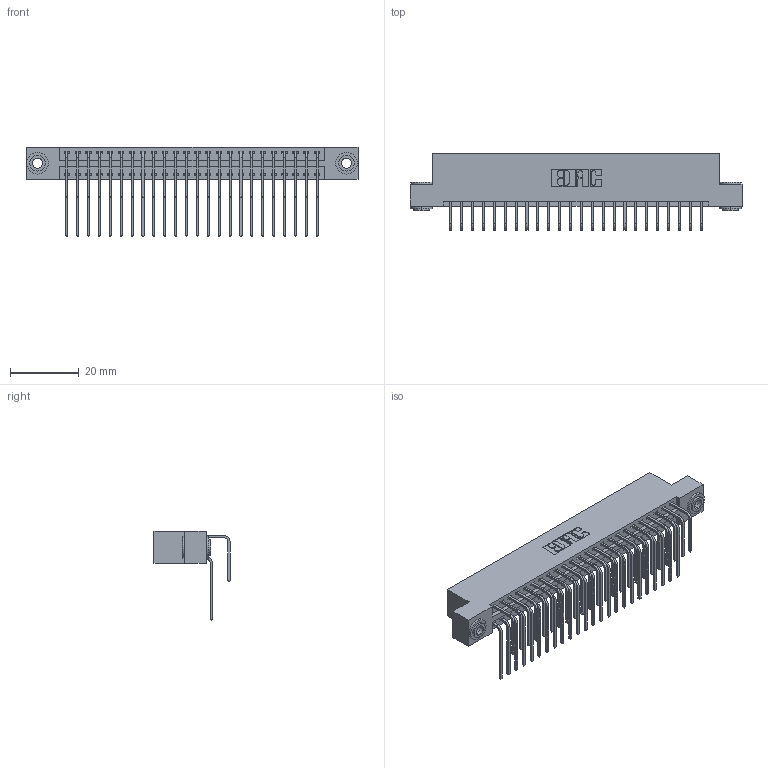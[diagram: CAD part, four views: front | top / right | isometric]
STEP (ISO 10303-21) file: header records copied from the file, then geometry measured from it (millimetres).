
FILE_DESCRIPTION (( 'STEP AP203' ), '1' );
FILE_NAME ('346-048-558-203.STEP', '2018-08-25T10:47:01', ( '' ), ( '' ), 'SwSTEP 2.0', 'SolidWorks 2016', '' );
FILE_SCHEMA (( 'CONFIG_CONTROL_DESIGN' ));
Length unit declared in the file: inch
Products named in the file (5): 346 Part_Flush Mounting Lugs - 0.156 Dia-TH; 345-292-001_558 559 Tail - 1; 345-292-001_558 Tail - 2; 345-250-002_345-250-002-102; 346-048-558-203
Assembly tree (51 placements, depth 2):
  346-048-558-203
    346 Part_Flush Mounting Lugs - 0.156 Dia-TH
    345-292-001_558 559 Tail - 1  x24
    345-292-001_558 Tail - 2  x24
    345-250-002_345-250-002-102  x2
Bounding box: 96.77 x 22.16 x 26.16 mm (x, y, z)
Volume: 9593.2 mm3; surface area: 14446.1 mm2
Topology: 51 solids, 51 shells, 2752 faces, 8133 edges, 5354 vertices
Faces by surface type: plane 1862, cylinder 882, cone 8
Entity records: 20520 total; most frequent: CARTESIAN_POINT 3434, ORIENTED_EDGE 3310, DIRECTION 3081, EDGE_CURVE 1655, VECTOR 1363, LINE 1363, VERTEX_POINT 1098, AXIS2_PLACEMENT_3D 859
